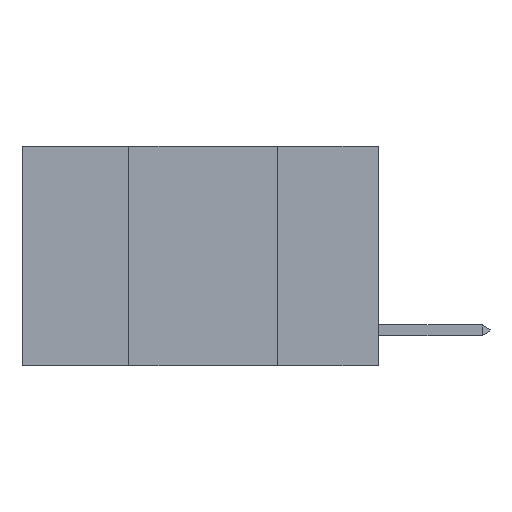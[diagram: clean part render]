
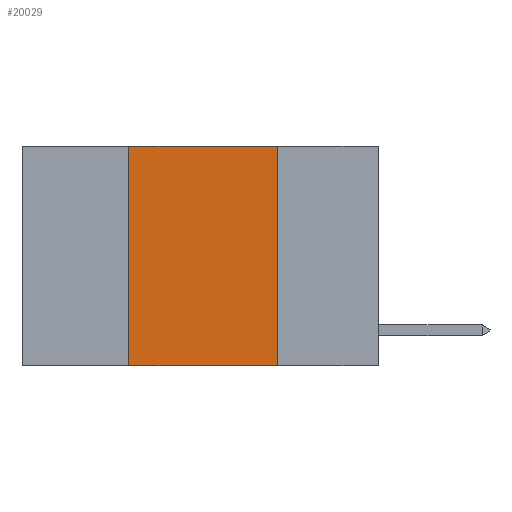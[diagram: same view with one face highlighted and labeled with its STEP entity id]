
A CAD part, left-side view. The second image highlights one B-rep face of the part: STEP entity #20029.
In plain terms, the highlighted planar face has unit normal (-1, 0, 0).
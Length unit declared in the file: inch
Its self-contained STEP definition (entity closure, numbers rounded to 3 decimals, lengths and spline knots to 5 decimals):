
#2794 = VECTOR ( 'NONE', #7891, 39.37008 ) ;
#2996 = AXIS2_PLACEMENT_3D ( 'NONE', #4185, #10432, #24392 ) ;
#3061 = VERTEX_POINT ( 'NONE', #25776 ) ;
#3669 = EDGE_CURVE ( 'NONE', #20505, #3061, #20724, .T. ) ;
#4185 = CARTESIAN_POINT ( 'NONE',  ( 0., 0.6, 0. ) ) ;
#4357 = VERTEX_POINT ( 'NONE', #13508 ) ;
#4445 = ORIENTED_EDGE ( 'NONE', *, *, #23838, .F. ) ;
#4819 = DIRECTION ( 'NONE',  ( 0., -1., 0. ) ) ;
#4904 = CARTESIAN_POINT ( 'NONE',  ( 0., 0.6, 0. ) ) ;
#5820 = CARTESIAN_POINT ( 'NONE',  ( 0., 0.42, 0. ) ) ;
#6405 = ORIENTED_EDGE ( 'NONE', *, *, #6489, .F. ) ;
#6489 = EDGE_CURVE ( 'NONE', #20505, #4357, #19035, .T. ) ;
#7891 = DIRECTION ( 'NONE',  ( 0., 0., 1. ) ) ;
#8699 = EDGE_LOOP ( 'NONE', ( #21049, #4445, #6405, #25512 ) ) ;
#9245 = EDGE_CURVE ( 'NONE', #13322, #3061, #23275, .T. ) ;
#9623 = DIRECTION ( 'NONE',  ( 0., 0., -1. ) ) ;
#10067 = VECTOR ( 'NONE', #19011, 39.37008 ) ;
#10432 = DIRECTION ( 'NONE',  ( 1., 0., 0. ) ) ;
#12050 = VECTOR ( 'NONE', #9623, 39.37008 ) ;
#12389 = PLANE ( 'NONE',  #2996 ) ;
#13322 = VERTEX_POINT ( 'NONE', #19782 ) ;
#13508 = CARTESIAN_POINT ( 'NONE',  ( 0., 0.42, 0. ) ) ;
#13845 = CARTESIAN_POINT ( 'NONE',  ( 0., 0.42, -0.37 ) ) ;
#16997 = CARTESIAN_POINT ( 'NONE',  ( 0., 0.6, -0.37 ) ) ;
#19011 = DIRECTION ( 'NONE',  ( 0., -1., 0. ) ) ;
#19035 = LINE ( 'NONE', #5820, #2794 ) ;
#19604 = CARTESIAN_POINT ( 'NONE',  ( 0., 0.17, 0. ) ) ;
#19782 = CARTESIAN_POINT ( 'NONE',  ( 0., 0.17, 0. ) ) ;
#20029 = ADVANCED_FACE ( 'NONE', ( #25738 ), #12389, .F. ) ;
#20505 = VERTEX_POINT ( 'NONE', #13845 ) ;
#20724 = LINE ( 'NONE', #16997, #10067 ) ;
#21049 = ORIENTED_EDGE ( 'NONE', *, *, #9245, .F. ) ;
#22749 = LINE ( 'NONE', #4904, #24589 ) ;
#23275 = LINE ( 'NONE', #19604, #12050 ) ;
#23838 = EDGE_CURVE ( 'NONE', #4357, #13322, #22749, .T. ) ;
#24392 = DIRECTION ( 'NONE',  ( 0., 0., -1. ) ) ;
#24589 = VECTOR ( 'NONE', #4819, 39.37008 ) ;
#25512 = ORIENTED_EDGE ( 'NONE', *, *, #3669, .T. ) ;
#25738 = FACE_OUTER_BOUND ( 'NONE', #8699, .T. ) ;
#25776 = CARTESIAN_POINT ( 'NONE',  ( 0., 0.17, -0.37 ) ) ;
